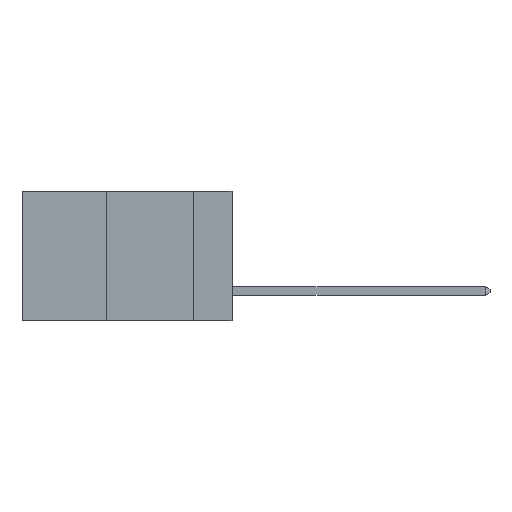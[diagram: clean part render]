
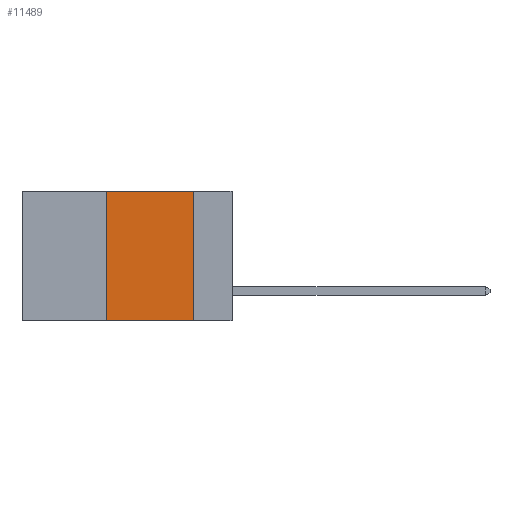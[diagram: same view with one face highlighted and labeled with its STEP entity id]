
A CAD part, left-side view. The second image highlights one B-rep face of the part: STEP entity #11489.
In plain terms, the highlighted planar face has unit normal (-1, 0, 0).
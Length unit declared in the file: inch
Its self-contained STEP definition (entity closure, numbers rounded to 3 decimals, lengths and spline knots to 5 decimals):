
#165 = DIRECTION ( 'NONE',  ( 0., 0., -1. ) ) ;
#234 = DIRECTION ( 'NONE',  ( 0., 0., 1. ) ) ;
#294 = EDGE_CURVE ( 'NONE', #2865, #13008, #17125, .T. ) ;
#1003 = ORIENTED_EDGE ( 'NONE', *, *, #14767, .F. ) ;
#1012 = CARTESIAN_POINT ( 'NONE',  ( 0., 0.6, 0. ) ) ;
#1115 = CARTESIAN_POINT ( 'NONE',  ( 0., 0.36, 0. ) ) ;
#2122 = AXIS2_PLACEMENT_3D ( 'NONE', #18171, #9409, #165 ) ;
#2331 = CARTESIAN_POINT ( 'NONE',  ( 0., 0.11, 0. ) ) ;
#2549 = DIRECTION ( 'NONE',  ( 0., -1., 0. ) ) ;
#2865 = VERTEX_POINT ( 'NONE', #14809 ) ;
#2986 = DIRECTION ( 'NONE',  ( 0., 0., -1. ) ) ;
#3664 = VECTOR ( 'NONE', #2549, 39.37008 ) ;
#5559 = CARTESIAN_POINT ( 'NONE',  ( 0., 0.6, -0.37 ) ) ;
#6127 = ORIENTED_EDGE ( 'NONE', *, *, #11516, .F. ) ;
#6414 = DIRECTION ( 'NONE',  ( 0., -1., 0. ) ) ;
#6766 = VERTEX_POINT ( 'NONE', #2331 ) ;
#7887 = FACE_OUTER_BOUND ( 'NONE', #8026, .T. ) ;
#8026 = EDGE_LOOP ( 'NONE', ( #16584, #1003, #6127, #16368 ) ) ;
#8634 = CARTESIAN_POINT ( 'NONE',  ( 0., 0.11, -0.37 ) ) ;
#9409 = DIRECTION ( 'NONE',  ( 1., 0., 0. ) ) ;
#11489 = ADVANCED_FACE ( 'NONE', ( #7887 ), #16738, .F. ) ;
#11516 = EDGE_CURVE ( 'NONE', #2865, #15410, #15346, .T. ) ;
#12278 = LINE ( 'NONE', #1012, #3664 ) ;
#13008 = VERTEX_POINT ( 'NONE', #8634 ) ;
#13676 = CARTESIAN_POINT ( 'NONE',  ( 0., 0.11, 0. ) ) ;
#13726 = LINE ( 'NONE', #13676, #17048 ) ;
#13849 = EDGE_CURVE ( 'NONE', #6766, #13008, #13726, .T. ) ;
#13955 = CARTESIAN_POINT ( 'NONE',  ( 0., 0.36, 0. ) ) ;
#14767 = EDGE_CURVE ( 'NONE', #15410, #6766, #12278, .T. ) ;
#14809 = CARTESIAN_POINT ( 'NONE',  ( 0., 0.36, -0.37 ) ) ;
#14914 = VECTOR ( 'NONE', #234, 39.37008 ) ;
#15346 = LINE ( 'NONE', #13955, #14914 ) ;
#15410 = VERTEX_POINT ( 'NONE', #1115 ) ;
#16368 = ORIENTED_EDGE ( 'NONE', *, *, #294, .T. ) ;
#16584 = ORIENTED_EDGE ( 'NONE', *, *, #13849, .F. ) ;
#16691 = VECTOR ( 'NONE', #6414, 39.37008 ) ;
#16738 = PLANE ( 'NONE',  #2122 ) ;
#17048 = VECTOR ( 'NONE', #2986, 39.37008 ) ;
#17125 = LINE ( 'NONE', #5559, #16691 ) ;
#18171 = CARTESIAN_POINT ( 'NONE',  ( 0., 0.6, 0. ) ) ;
